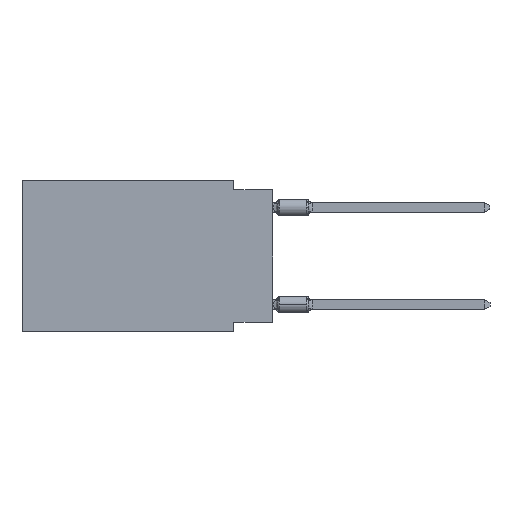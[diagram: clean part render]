
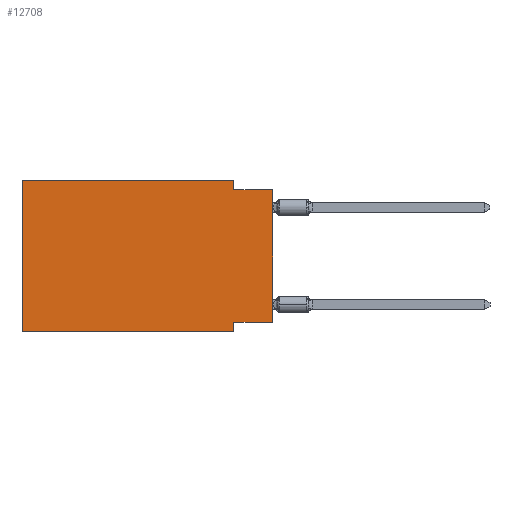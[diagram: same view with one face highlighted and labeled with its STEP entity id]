
A CAD part, left-side view. The second image highlights one B-rep face of the part: STEP entity #12708.
In plain terms, the highlighted planar face has unit normal (-1, 0, 0).
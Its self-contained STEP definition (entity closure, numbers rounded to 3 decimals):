
#513 = EDGE_CURVE ( 'NONE', #17368, #19721, #22885, .T. ) ;
#869 = CARTESIAN_POINT ( 'NONE',  ( 0., 16.383, 0. ) ) ;
#1002 = DIRECTION ( 'NONE',  ( 0., 0., 1. ) ) ;
#1230 = VECTOR ( 'NONE', #25586, 1000. ) ;
#2068 = EDGE_CURVE ( 'NONE', #23260, #4025, #18281, .T. ) ;
#2186 = DIRECTION ( 'NONE',  ( 1., 0., 0. ) ) ;
#2724 = CARTESIAN_POINT ( 'NONE',  ( 0., 2.54, 0. ) ) ;
#2997 = ORIENTED_EDGE ( 'NONE', *, *, #25410, .F. ) ;
#4025 = VERTEX_POINT ( 'NONE', #17968 ) ;
#4111 = LINE ( 'NONE', #10256, #4567 ) ;
#4282 = VECTOR ( 'NONE', #11578, 1000. ) ;
#4361 = CARTESIAN_POINT ( 'NONE',  ( 0., 2.54, -0.635 ) ) ;
#4567 = VECTOR ( 'NONE', #23492, 1000. ) ;
#4575 = ORIENTED_EDGE ( 'NONE', *, *, #14385, .T. ) ;
#4604 = CARTESIAN_POINT ( 'NONE',  ( 0., 2.54, -9.271 ) ) ;
#4703 = VERTEX_POINT ( 'NONE', #11965 ) ;
#5139 = DIRECTION ( 'NONE',  ( 0., 0., -1. ) ) ;
#6246 = VERTEX_POINT ( 'NONE', #21931 ) ;
#9059 = FACE_OUTER_BOUND ( 'NONE', #10730, .T. ) ;
#9452 = VECTOR ( 'NONE', #5139, 1000. ) ;
#9868 = LINE ( 'NONE', #869, #24799 ) ;
#9908 = DIRECTION ( 'NONE',  ( 0., -1., 0. ) ) ;
#10200 = LINE ( 'NONE', #23435, #1230 ) ;
#10208 = DIRECTION ( 'NONE',  ( 0., 0., -1. ) ) ;
#10223 = EDGE_CURVE ( 'NONE', #6246, #23260, #9868, .T. ) ;
#10256 = CARTESIAN_POINT ( 'NONE',  ( 0., 16.383, -9.906 ) ) ;
#10266 = DIRECTION ( 'NONE',  ( 0., -1., 0. ) ) ;
#10339 = VECTOR ( 'NONE', #10208, 1000. ) ;
#10483 = VERTEX_POINT ( 'NONE', #14302 ) ;
#10634 = DIRECTION ( 'NONE',  ( 0., 0., -1. ) ) ;
#10730 = EDGE_LOOP ( 'NONE', ( #4575, #2997, #20758, #11132, #13029, #19787, #27875, #10860 ) ) ;
#10860 = ORIENTED_EDGE ( 'NONE', *, *, #18587, .F. ) ;
#11132 = ORIENTED_EDGE ( 'NONE', *, *, #2068, .F. ) ;
#11578 = DIRECTION ( 'NONE',  ( 0., 1., 0. ) ) ;
#11843 = CARTESIAN_POINT ( 'NONE',  ( 0., 0., -9.271 ) ) ;
#11965 = CARTESIAN_POINT ( 'NONE',  ( 0., 0., -9.271 ) ) ;
#12708 = ADVANCED_FACE ( 'NONE', ( #9059 ), #21699, .F. ) ;
#13029 = ORIENTED_EDGE ( 'NONE', *, *, #10223, .F. ) ;
#14007 = LINE ( 'NONE', #11843, #4282 ) ;
#14249 = CARTESIAN_POINT ( 'NONE',  ( 0., 2.54, -9.906 ) ) ;
#14302 = CARTESIAN_POINT ( 'NONE',  ( 0., 0., -0.635 ) ) ;
#14385 = EDGE_CURVE ( 'NONE', #4703, #10483, #10200, .T. ) ;
#17368 = VERTEX_POINT ( 'NONE', #4604 ) ;
#17968 = CARTESIAN_POINT ( 'NONE',  ( 0., 2.54, 0. ) ) ;
#18281 = LINE ( 'NONE', #18411, #27387 ) ;
#18339 = LINE ( 'NONE', #2724, #9452 ) ;
#18411 = CARTESIAN_POINT ( 'NONE',  ( 0., 16.383, 0. ) ) ;
#18587 = EDGE_CURVE ( 'NONE', #4703, #17368, #14007, .T. ) ;
#18900 = LINE ( 'NONE', #21047, #22762 ) ;
#19688 = CARTESIAN_POINT ( 'NONE',  ( 0., 16.383, 0. ) ) ;
#19721 = VERTEX_POINT ( 'NONE', #22680 ) ;
#19787 = ORIENTED_EDGE ( 'NONE', *, *, #23809, .T. ) ;
#20547 = CARTESIAN_POINT ( 'NONE',  ( 0., 16.383, 0. ) ) ;
#20758 = ORIENTED_EDGE ( 'NONE', *, *, #21326, .F. ) ;
#21047 = CARTESIAN_POINT ( 'NONE',  ( 0., 0., -0.635 ) ) ;
#21326 = EDGE_CURVE ( 'NONE', #4025, #24371, #18339, .T. ) ;
#21699 = PLANE ( 'NONE',  #28205 ) ;
#21931 = CARTESIAN_POINT ( 'NONE',  ( 0., 16.383, -9.906 ) ) ;
#22680 = CARTESIAN_POINT ( 'NONE',  ( 0., 2.54, -9.906 ) ) ;
#22762 = VECTOR ( 'NONE', #10266, 1000. ) ;
#22885 = LINE ( 'NONE', #14249, #10339 ) ;
#23260 = VERTEX_POINT ( 'NONE', #20547 ) ;
#23435 = CARTESIAN_POINT ( 'NONE',  ( 0., 0., 0. ) ) ;
#23492 = DIRECTION ( 'NONE',  ( 0., -1., 0. ) ) ;
#23809 = EDGE_CURVE ( 'NONE', #6246, #19721, #4111, .T. ) ;
#24371 = VERTEX_POINT ( 'NONE', #4361 ) ;
#24799 = VECTOR ( 'NONE', #1002, 1000. ) ;
#25410 = EDGE_CURVE ( 'NONE', #24371, #10483, #18900, .T. ) ;
#25586 = DIRECTION ( 'NONE',  ( 0., 0., 1. ) ) ;
#27387 = VECTOR ( 'NONE', #9908, 1000. ) ;
#27875 = ORIENTED_EDGE ( 'NONE', *, *, #513, .F. ) ;
#28205 = AXIS2_PLACEMENT_3D ( 'NONE', #19688, #2186, #10634 ) ;
